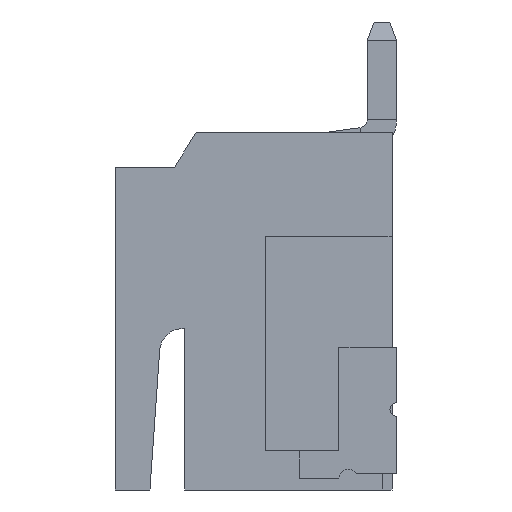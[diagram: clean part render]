
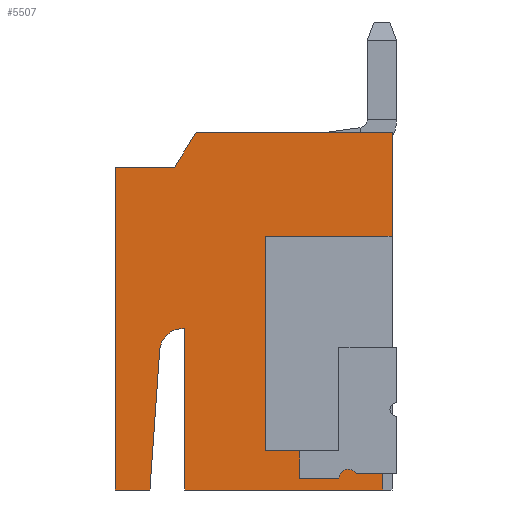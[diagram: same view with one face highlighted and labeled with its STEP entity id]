
A CAD part, left-side view. The second image highlights one B-rep face of the part: STEP entity #5507.
In plain terms, the highlighted planar face has unit normal (-1, 0, 0).
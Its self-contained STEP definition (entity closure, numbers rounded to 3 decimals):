
#30 = CARTESIAN_POINT ( 'NONE',  ( -21.25, -2.9, -3.875 ) ) ;
#81 = VECTOR ( 'NONE', #8743, 1000. ) ;
#92 = VECTOR ( 'NONE', #12128, 1000. ) ;
#315 = AXIS2_PLACEMENT_3D ( 'NONE', #4655, #12467, #9193 ) ;
#321 = CARTESIAN_POINT ( 'NONE',  ( -21.25, -0.35, 1.625 ) ) ;
#426 = CARTESIAN_POINT ( 'NONE',  ( -21.25, -0.35, -3.025 ) ) ;
#429 = EDGE_CURVE ( 'NONE', #607, #6629, #2804, .T. ) ;
#535 = VECTOR ( 'NONE', #9946, 1000. ) ;
#607 = VERTEX_POINT ( 'NONE', #3668 ) ;
#686 = CARTESIAN_POINT ( 'NONE',  ( -21.25, 1.439, -0.873 ) ) ;
#775 = DIRECTION ( 'NONE',  ( 0., 0., 1. ) ) ;
#808 = ORIENTED_EDGE ( 'NONE', *, *, #7050, .F. ) ;
#914 = VERTEX_POINT ( 'NONE', #4579 ) ;
#978 = EDGE_CURVE ( 'NONE', #11326, #11305, #12655, .T. ) ;
#1009 = CARTESIAN_POINT ( 'NONE',  ( -21.25, -0.35, -3.025 ) ) ;
#1019 = VECTOR ( 'NONE', #3140, 1000. ) ;
#1050 = CARTESIAN_POINT ( 'NONE',  ( -21.25, -1.95, -3.625 ) ) ;
#1176 = VECTOR ( 'NONE', #1942, 1000. ) ;
#1187 = VERTEX_POINT ( 'NONE', #5010 ) ;
#1412 = VERTEX_POINT ( 'NONE', #3451 ) ;
#1473 = AXIS2_PLACEMENT_3D ( 'NONE', #5676, #7833, #10368 ) ;
#1517 = LINE ( 'NONE', #8433, #7656 ) ;
#1605 = VERTEX_POINT ( 'NONE', #4921 ) ;
#1631 = ORIENTED_EDGE ( 'NONE', *, *, #14256, .F. ) ;
#1751 = LINE ( 'NONE', #2796, #1822 ) ;
#1822 = VECTOR ( 'NONE', #775, 1000. ) ;
#1942 = DIRECTION ( 'NONE',  ( 0., 0., 1. ) ) ;
#2133 = EDGE_LOOP ( 'NONE', ( #6367, #6844, #13312, #4919, #8863, #9668, #12228, #11293, #9730, #7732, #9466, #13745, #14646, #3779, #1631, #808, #11532, #11653 ) ) ;
#2205 = VECTOR ( 'NONE', #2409, 1000. ) ;
#2344 = EDGE_CURVE ( 'NONE', #1187, #9565, #14014, .T. ) ;
#2362 = AXIS2_PLACEMENT_3D ( 'NONE', #686, #9910, #10055 ) ;
#2409 = DIRECTION ( 'NONE',  ( 0., 1., 0. ) ) ;
#2596 = CARTESIAN_POINT ( 'NONE',  ( -21.25, 1.4, -0.375 ) ) ;
#2736 = DIRECTION ( 'NONE',  ( 0., 1., 0. ) ) ;
#2796 = CARTESIAN_POINT ( 'NONE',  ( -21.25, -1.1, -0.775 ) ) ;
#2804 = LINE ( 'NONE', #426, #12402 ) ;
#2821 = EDGE_CURVE ( 'NONE', #6629, #1187, #10500, .T. ) ;
#2920 = LINE ( 'NONE', #6397, #1176 ) ;
#2958 = CARTESIAN_POINT ( 'NONE',  ( -21.25, -1.1, -3.625 ) ) ;
#3140 = DIRECTION ( 'NONE',  ( 0., 0., 1. ) ) ;
#3337 = CARTESIAN_POINT ( 'NONE',  ( -21.25, 1.938, -0.839 ) ) ;
#3451 = CARTESIAN_POINT ( 'NONE',  ( -21.25, 1.619, 3.125 ) ) ;
#3523 = VERTEX_POINT ( 'NONE', #3337 ) ;
#3668 = CARTESIAN_POINT ( 'NONE',  ( -21.25, -1.1, -3.025 ) ) ;
#3745 = VERTEX_POINT ( 'NONE', #2958 ) ;
#3779 = ORIENTED_EDGE ( 'NONE', *, *, #7252, .F. ) ;
#3864 = EDGE_CURVE ( 'NONE', #914, #10888, #5753, .T. ) ;
#4064 = EDGE_CURVE ( 'NONE', #11387, #8956, #1517, .T. ) ;
#4157 = LINE ( 'NONE', #9810, #13920 ) ;
#4450 = CARTESIAN_POINT ( 'NONE',  ( -21.25, -2.9, -3.875 ) ) ;
#4579 = CARTESIAN_POINT ( 'NONE',  ( -21.25, 2.15, -3.875 ) ) ;
#4640 = FACE_OUTER_BOUND ( 'NONE', #2133, .T. ) ;
#4655 = CARTESIAN_POINT ( 'NONE',  ( -21.25, -2.15, -3.625 ) ) ;
#4806 = VECTOR ( 'NONE', #13658, 1000. ) ;
#4829 = VERTEX_POINT ( 'NONE', #7335 ) ;
#4919 = ORIENTED_EDGE ( 'NONE', *, *, #11660, .F. ) ;
#4921 = CARTESIAN_POINT ( 'NONE',  ( -21.25, -2.9, -3.525 ) ) ;
#5010 = CARTESIAN_POINT ( 'NONE',  ( -21.25, -0.35, 1.625 ) ) ;
#5402 = LINE ( 'NONE', #12175, #535 ) ;
#5435 = DIRECTION ( 'NONE',  ( 0., 1., 0. ) ) ;
#5507 = ADVANCED_FACE ( 'NONE', ( #4640 ), #13701, .F. ) ;
#5676 = CARTESIAN_POINT ( 'NONE',  ( -21.25, 0., 0. ) ) ;
#5753 = LINE ( 'NONE', #30, #2205 ) ;
#5908 = VECTOR ( 'NONE', #5435, 1000. ) ;
#6367 = ORIENTED_EDGE ( 'NONE', *, *, #7067, .T. ) ;
#6397 = CARTESIAN_POINT ( 'NONE',  ( -21.25, 2.9, -3.875 ) ) ;
#6629 = VERTEX_POINT ( 'NONE', #1009 ) ;
#6841 = CARTESIAN_POINT ( 'NONE',  ( -21.25, 1.619, 3.125 ) ) ;
#6844 = ORIENTED_EDGE ( 'NONE', *, *, #4064, .T. ) ;
#7050 = EDGE_CURVE ( 'NONE', #10888, #8471, #2920, .T. ) ;
#7067 = EDGE_CURVE ( 'NONE', #3523, #11387, #8762, .T. ) ;
#7138 = CARTESIAN_POINT ( 'NONE',  ( -21.25, 2.9, -3.875 ) ) ;
#7144 = EDGE_CURVE ( 'NONE', #13650, #8956, #12209, .T. ) ;
#7252 = EDGE_CURVE ( 'NONE', #1412, #9229, #8108, .T. ) ;
#7308 = LINE ( 'NONE', #13243, #92 ) ;
#7319 = CARTESIAN_POINT ( 'NONE',  ( -21.25, -2.9, 1.625 ) ) ;
#7335 = CARTESIAN_POINT ( 'NONE',  ( -21.25, -3.1, 3.875 ) ) ;
#7656 = VECTOR ( 'NONE', #14004, 1000. ) ;
#7732 = ORIENTED_EDGE ( 'NONE', *, *, #2821, .T. ) ;
#7820 = DIRECTION ( 'NONE',  ( 0., -0.53, 0.848 ) ) ;
#7833 = DIRECTION ( 'NONE',  ( 1., 0., 0. ) ) ;
#8108 = LINE ( 'NONE', #6841, #13036 ) ;
#8290 = CARTESIAN_POINT ( 'NONE',  ( -21.25, 2.9, 3.125 ) ) ;
#8433 = CARTESIAN_POINT ( 'NONE',  ( -21.25, 1.4, 0. ) ) ;
#8471 = VERTEX_POINT ( 'NONE', #13397 ) ;
#8511 = DIRECTION ( 'NONE',  ( 0., -1., 0. ) ) ;
#8711 = EDGE_CURVE ( 'NONE', #1605, #11326, #4157, .T. ) ;
#8743 = DIRECTION ( 'NONE',  ( 0., 1., 0. ) ) ;
#8762 = CIRCLE ( 'NONE', #2362, 0.5 ) ;
#8789 = CARTESIAN_POINT ( 'NONE',  ( -21.25, -2.9, -3.875 ) ) ;
#8863 = ORIENTED_EDGE ( 'NONE', *, *, #8711, .T. ) ;
#8872 = VECTOR ( 'NONE', #12823, 1000. ) ;
#8956 = VERTEX_POINT ( 'NONE', #9563 ) ;
#8978 = EDGE_CURVE ( 'NONE', #3745, #607, #1751, .T. ) ;
#9193 = DIRECTION ( 'NONE',  ( 0., 0., -1. ) ) ;
#9203 = LINE ( 'NONE', #12395, #4806 ) ;
#9229 = VERTEX_POINT ( 'NONE', #13706 ) ;
#9399 = DIRECTION ( 'NONE',  ( 0., 0., 1. ) ) ;
#9466 = ORIENTED_EDGE ( 'NONE', *, *, #2344, .T. ) ;
#9563 = CARTESIAN_POINT ( 'NONE',  ( -21.25, 1.4, -3.875 ) ) ;
#9565 = VERTEX_POINT ( 'NONE', #13464 ) ;
#9668 = ORIENTED_EDGE ( 'NONE', *, *, #978, .T. ) ;
#9730 = ORIENTED_EDGE ( 'NONE', *, *, #429, .T. ) ;
#9810 = CARTESIAN_POINT ( 'NONE',  ( -21.25, -2.323, -3.525 ) ) ;
#9861 = LINE ( 'NONE', #13417, #81 ) ;
#9910 = DIRECTION ( 'NONE',  ( 1., 0., 0. ) ) ;
#9946 = DIRECTION ( 'NONE',  ( 0., 0., -1. ) ) ;
#10055 = DIRECTION ( 'NONE',  ( 0., 0., -1. ) ) ;
#10368 = DIRECTION ( 'NONE',  ( 0., 0., -1. ) ) ;
#10500 = LINE ( 'NONE', #321, #13382 ) ;
#10888 = VERTEX_POINT ( 'NONE', #7138 ) ;
#11064 = DIRECTION ( 'NONE',  ( 0., 1., 0. ) ) ;
#11293 = ORIENTED_EDGE ( 'NONE', *, *, #8978, .T. ) ;
#11305 = VERTEX_POINT ( 'NONE', #1050 ) ;
#11326 = VERTEX_POINT ( 'NONE', #13671 ) ;
#11387 = VERTEX_POINT ( 'NONE', #2596 ) ;
#11532 = ORIENTED_EDGE ( 'NONE', *, *, #3864, .F. ) ;
#11653 = ORIENTED_EDGE ( 'NONE', *, *, #11780, .T. ) ;
#11660 = EDGE_CURVE ( 'NONE', #1605, #13650, #5402, .T. ) ;
#11780 = EDGE_CURVE ( 'NONE', #914, #3523, #9203, .T. ) ;
#11998 = EDGE_CURVE ( 'NONE', #9565, #4829, #14443, .T. ) ;
#12128 = DIRECTION ( 'NONE',  ( 0., -1., 0. ) ) ;
#12175 = CARTESIAN_POINT ( 'NONE',  ( -21.25, -2.9, 3.875 ) ) ;
#12209 = LINE ( 'NONE', #8789, #5908 ) ;
#12228 = ORIENTED_EDGE ( 'NONE', *, *, #13901, .T. ) ;
#12395 = CARTESIAN_POINT ( 'NONE',  ( -21.25, 1.87, 0.131 ) ) ;
#12402 = VECTOR ( 'NONE', #2736, 1000. ) ;
#12467 = DIRECTION ( 'NONE',  ( -1., 0., 0. ) ) ;
#12516 = CARTESIAN_POINT ( 'NONE',  ( -21.25, -3.1, 3.875 ) ) ;
#12655 = CIRCLE ( 'NONE', #315, 0.2 ) ;
#12823 = DIRECTION ( 'NONE',  ( 0., -1., 0. ) ) ;
#12919 = VECTOR ( 'NONE', #8511, 1000. ) ;
#13036 = VECTOR ( 'NONE', #7820, 1000. ) ;
#13162 = EDGE_CURVE ( 'NONE', #9229, #4829, #7308, .T. ) ;
#13243 = CARTESIAN_POINT ( 'NONE',  ( -21.25, 1.15, 3.875 ) ) ;
#13312 = ORIENTED_EDGE ( 'NONE', *, *, #7144, .F. ) ;
#13382 = VECTOR ( 'NONE', #9399, 1000. ) ;
#13397 = CARTESIAN_POINT ( 'NONE',  ( -21.25, 2.9, 3.125 ) ) ;
#13417 = CARTESIAN_POINT ( 'NONE',  ( -21.25, -1.1, -3.625 ) ) ;
#13464 = CARTESIAN_POINT ( 'NONE',  ( -21.25, -3.1, 1.625 ) ) ;
#13650 = VERTEX_POINT ( 'NONE', #4450 ) ;
#13658 = DIRECTION ( 'NONE',  ( 0., -0.07, 0.998 ) ) ;
#13671 = CARTESIAN_POINT ( 'NONE',  ( -21.25, -2.323, -3.525 ) ) ;
#13701 = PLANE ( 'NONE',  #1473 ) ;
#13706 = CARTESIAN_POINT ( 'NONE',  ( -21.25, 1.15, 3.875 ) ) ;
#13745 = ORIENTED_EDGE ( 'NONE', *, *, #11998, .T. ) ;
#13901 = EDGE_CURVE ( 'NONE', #11305, #3745, #9861, .T. ) ;
#13920 = VECTOR ( 'NONE', #11064, 1000. ) ;
#14004 = DIRECTION ( 'NONE',  ( 0., 0., -1. ) ) ;
#14014 = LINE ( 'NONE', #7319, #12919 ) ;
#14085 = LINE ( 'NONE', #8290, #8872 ) ;
#14256 = EDGE_CURVE ( 'NONE', #8471, #1412, #14085, .T. ) ;
#14443 = LINE ( 'NONE', #12516, #1019 ) ;
#14646 = ORIENTED_EDGE ( 'NONE', *, *, #13162, .F. ) ;
